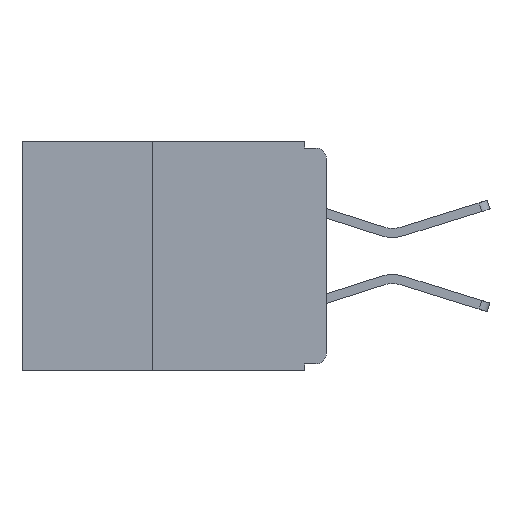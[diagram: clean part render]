
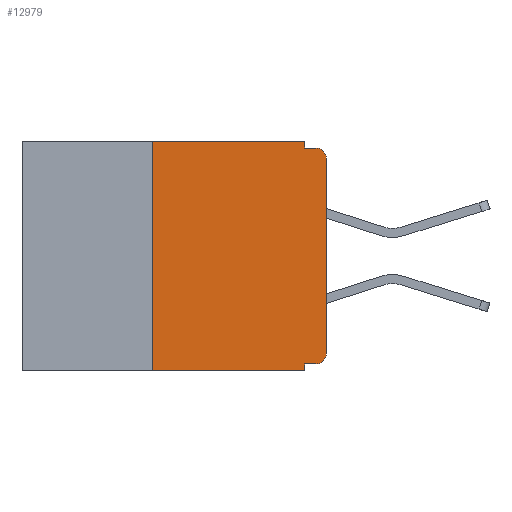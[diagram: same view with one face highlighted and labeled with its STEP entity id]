
A CAD part, left-side view. The second image highlights one B-rep face of the part: STEP entity #12979.
In plain terms, the highlighted planar face has unit normal (-1, 0, 0).
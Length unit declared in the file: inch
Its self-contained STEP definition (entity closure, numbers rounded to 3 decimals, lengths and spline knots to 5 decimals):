
#91 = DIRECTION ( 'NONE',  ( 0., 0., 1. ) ) ;
#177 = DIRECTION ( 'NONE',  ( 0., 0., -1. ) ) ;
#439 = LINE ( 'NONE', #24384, #6610 ) ;
#1655 = CARTESIAN_POINT ( 'NONE',  ( 0., 0.25, 0. ) ) ;
#3744 = LINE ( 'NONE', #25462, #23893 ) ;
#5148 = CARTESIAN_POINT ( 'NONE',  ( 0., 0., -0.32 ) ) ;
#5194 = CARTESIAN_POINT ( 'NONE',  ( 0., 0.031, -0.33 ) ) ;
#5400 = EDGE_CURVE ( 'NONE', #16533, #19140, #6293, .T. ) ;
#5430 = CARTESIAN_POINT ( 'NONE',  ( 0., 0., -0.305 ) ) ;
#5731 = VERTEX_POINT ( 'NONE', #9152 ) ;
#5835 = VERTEX_POINT ( 'NONE', #1655 ) ;
#6293 = LINE ( 'NONE', #5148, #19443 ) ;
#6454 = EDGE_CURVE ( 'NONE', #11496, #5835, #16859, .T. ) ;
#6521 = CIRCLE ( 'NONE', #27153, 0.015 ) ;
#6574 = EDGE_CURVE ( 'NONE', #19140, #21453, #11942, .T. ) ;
#6610 = VECTOR ( 'NONE', #11380, 39.37008 ) ;
#7077 = ORIENTED_EDGE ( 'NONE', *, *, #24748, .T. ) ;
#7271 = CARTESIAN_POINT ( 'NONE',  ( 0., 0.25, -0.33 ) ) ;
#7847 = DIRECTION ( 'NONE',  ( 0., 0., -1. ) ) ;
#8367 = EDGE_CURVE ( 'NONE', #5731, #26935, #31447, .T. ) ;
#8888 = VECTOR ( 'NONE', #91, 39.37008 ) ;
#9152 = CARTESIAN_POINT ( 'NONE',  ( 0., 0.031, -0.01 ) ) ;
#9816 = CARTESIAN_POINT ( 'NONE',  ( 0., 0.437, -0.33 ) ) ;
#10030 = CARTESIAN_POINT ( 'NONE',  ( 0., 0.031, 0. ) ) ;
#10127 = DIRECTION ( 'NONE',  ( 0., -1., 0. ) ) ;
#10306 = ORIENTED_EDGE ( 'NONE', *, *, #21937, .T. ) ;
#11209 = CARTESIAN_POINT ( 'NONE',  ( 0., 0.031, -0.33 ) ) ;
#11225 = ORIENTED_EDGE ( 'NONE', *, *, #11344, .T. ) ;
#11344 = EDGE_CURVE ( 'NONE', #16533, #19465, #23085, .T. ) ;
#11380 = DIRECTION ( 'NONE',  ( 0., 0., -1. ) ) ;
#11496 = VERTEX_POINT ( 'NONE', #29523 ) ;
#11942 = LINE ( 'NONE', #5194, #31922 ) ;
#12479 = DIRECTION ( 'NONE',  ( 0., -1., 0. ) ) ;
#12922 = EDGE_CURVE ( 'NONE', #5835, #18027, #3744, .T. ) ;
#12979 = ADVANCED_FACE ( 'NONE', ( #20612 ), #30908, .F. ) ;
#13253 = CARTESIAN_POINT ( 'NONE',  ( 0., 0., 0. ) ) ;
#13614 = ORIENTED_EDGE ( 'NONE', *, *, #20230, .T. ) ;
#13709 = DIRECTION ( 'NONE',  ( -1., 0., 0. ) ) ;
#15680 = ORIENTED_EDGE ( 'NONE', *, *, #8367, .F. ) ;
#15977 = DIRECTION ( 'NONE',  ( -1., 0., 0. ) ) ;
#16533 = VERTEX_POINT ( 'NONE', #17996 ) ;
#16859 = LINE ( 'NONE', #7271, #22132 ) ;
#17846 = DIRECTION ( 'NONE',  ( 0., 0., 1. ) ) ;
#17996 = CARTESIAN_POINT ( 'NONE',  ( 0., 0.015, -0.32 ) ) ;
#18027 = VERTEX_POINT ( 'NONE', #10030 ) ;
#18035 = DIRECTION ( 'NONE',  ( 0., 0., -1. ) ) ;
#18129 = ORIENTED_EDGE ( 'NONE', *, *, #29060, .F. ) ;
#18571 = ORIENTED_EDGE ( 'NONE', *, *, #6454, .F. ) ;
#18804 = VECTOR ( 'NONE', #12479, 39.37008 ) ;
#19140 = VERTEX_POINT ( 'NONE', #27687 ) ;
#19169 = AXIS2_PLACEMENT_3D ( 'NONE', #28441, #33561, #18035 ) ;
#19443 = VECTOR ( 'NONE', #26024, 39.37008 ) ;
#19465 = VERTEX_POINT ( 'NONE', #5430 ) ;
#20230 = EDGE_CURVE ( 'NONE', #22709, #26935, #6521, .T. ) ;
#20612 = FACE_OUTER_BOUND ( 'NONE', #32537, .T. ) ;
#21453 = VERTEX_POINT ( 'NONE', #11209 ) ;
#21937 = EDGE_CURVE ( 'NONE', #19465, #22709, #23644, .T. ) ;
#22132 = VECTOR ( 'NONE', #17846, 39.37008 ) ;
#22709 = VERTEX_POINT ( 'NONE', #32486 ) ;
#23080 = AXIS2_PLACEMENT_3D ( 'NONE', #31565, #15977, #177 ) ;
#23085 = CIRCLE ( 'NONE', #23080, 0.015 ) ;
#23147 = CARTESIAN_POINT ( 'NONE',  ( 0., 0.015, -0.01 ) ) ;
#23644 = LINE ( 'NONE', #13253, #8888 ) ;
#23893 = VECTOR ( 'NONE', #33241, 39.37008 ) ;
#24384 = CARTESIAN_POINT ( 'NONE',  ( 0., 0.031, 0. ) ) ;
#24748 = EDGE_CURVE ( 'NONE', #11496, #21453, #26599, .T. ) ;
#25462 = CARTESIAN_POINT ( 'NONE',  ( 0., 0.437, 0. ) ) ;
#25810 = CARTESIAN_POINT ( 'NONE',  ( 0., 0., -0.01 ) ) ;
#26024 = DIRECTION ( 'NONE',  ( 0., 1., 0. ) ) ;
#26335 = ORIENTED_EDGE ( 'NONE', *, *, #12922, .F. ) ;
#26599 = LINE ( 'NONE', #9816, #18804 ) ;
#26935 = VERTEX_POINT ( 'NONE', #23147 ) ;
#27153 = AXIS2_PLACEMENT_3D ( 'NONE', #29331, #13709, #31914 ) ;
#27687 = CARTESIAN_POINT ( 'NONE',  ( 0., 0.031, -0.32 ) ) ;
#28007 = ORIENTED_EDGE ( 'NONE', *, *, #6574, .F. ) ;
#28441 = CARTESIAN_POINT ( 'NONE',  ( 0., 0.437, 0. ) ) ;
#29060 = EDGE_CURVE ( 'NONE', #18027, #5731, #439, .T. ) ;
#29331 = CARTESIAN_POINT ( 'NONE',  ( 0., 0.015, -0.025 ) ) ;
#29523 = CARTESIAN_POINT ( 'NONE',  ( 0., 0.25, -0.33 ) ) ;
#29599 = ORIENTED_EDGE ( 'NONE', *, *, #5400, .F. ) ;
#30908 = PLANE ( 'NONE',  #19169 ) ;
#31447 = LINE ( 'NONE', #25810, #32226 ) ;
#31565 = CARTESIAN_POINT ( 'NONE',  ( 0., 0.015, -0.305 ) ) ;
#31914 = DIRECTION ( 'NONE',  ( 0., 0., -1. ) ) ;
#31922 = VECTOR ( 'NONE', #7847, 39.37008 ) ;
#32226 = VECTOR ( 'NONE', #10127, 39.37008 ) ;
#32486 = CARTESIAN_POINT ( 'NONE',  ( 0., 0., -0.025 ) ) ;
#32537 = EDGE_LOOP ( 'NONE', ( #10306, #13614, #15680, #18129, #26335, #18571, #7077, #28007, #29599, #11225 ) ) ;
#33241 = DIRECTION ( 'NONE',  ( 0., -1., 0. ) ) ;
#33561 = DIRECTION ( 'NONE',  ( 1., 0., 0. ) ) ;
